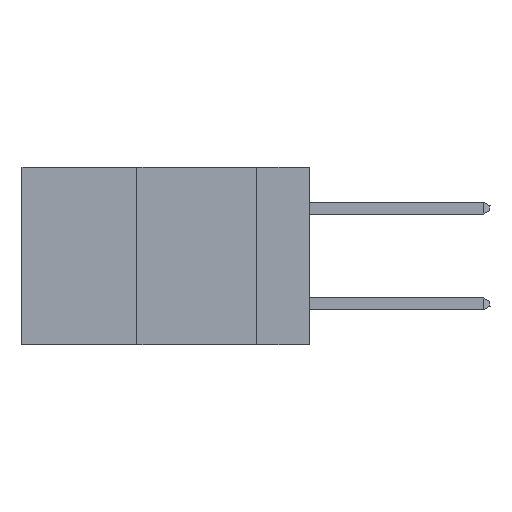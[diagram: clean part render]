
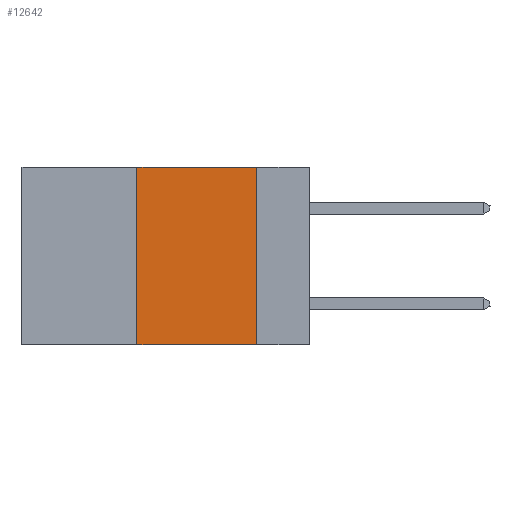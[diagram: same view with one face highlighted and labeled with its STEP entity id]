
A CAD part, left-side view. The second image highlights one B-rep face of the part: STEP entity #12642.
In plain terms, the highlighted planar face has unit normal (-1, 0, 0).
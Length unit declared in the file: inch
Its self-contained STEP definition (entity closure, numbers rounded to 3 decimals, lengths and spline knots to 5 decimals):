
#88 = CARTESIAN_POINT ( 'NONE',  ( 0., 0.36, 0. ) ) ;
#527 = CARTESIAN_POINT ( 'NONE',  ( 0., 0.6, 0. ) ) ;
#921 = LINE ( 'NONE', #35622, #24364 ) ;
#1566 = CARTESIAN_POINT ( 'NONE',  ( 0., 0.11, 0. ) ) ;
#4263 = EDGE_CURVE ( 'NONE', #24879, #12656, #921, .T. ) ;
#5585 = VECTOR ( 'NONE', #17706, 39.37008 ) ;
#6544 = LINE ( 'NONE', #11686, #5585 ) ;
#6609 = DIRECTION ( 'NONE',  ( 1., 0., 0. ) ) ;
#8636 = CARTESIAN_POINT ( 'NONE',  ( 0., 0.36, -0.37 ) ) ;
#8836 = LINE ( 'NONE', #35312, #28058 ) ;
#9610 = DIRECTION ( 'NONE',  ( 0., 0., -1. ) ) ;
#10953 = EDGE_CURVE ( 'NONE', #33151, #12656, #8836, .T. ) ;
#11686 = CARTESIAN_POINT ( 'NONE',  ( 0., 0.36, 0. ) ) ;
#11842 = ORIENTED_EDGE ( 'NONE', *, *, #33914, .F. ) ;
#12642 = ADVANCED_FACE ( 'NONE', ( #20418 ), #33520, .F. ) ;
#12656 = VERTEX_POINT ( 'NONE', #30481 ) ;
#14429 = DIRECTION ( 'NONE',  ( 0., -1., 0. ) ) ;
#15804 = VECTOR ( 'NONE', #14429, 39.37008 ) ;
#15939 = VERTEX_POINT ( 'NONE', #88 ) ;
#16555 = EDGE_CURVE ( 'NONE', #15939, #24879, #24757, .T. ) ;
#17706 = DIRECTION ( 'NONE',  ( 0., 0., 1. ) ) ;
#20418 = FACE_OUTER_BOUND ( 'NONE', #22758, .T. ) ;
#22758 = EDGE_LOOP ( 'NONE', ( #26031, #26876, #11842, #29586 ) ) ;
#24204 = DIRECTION ( 'NONE',  ( 0., -1., 0. ) ) ;
#24364 = VECTOR ( 'NONE', #29298, 39.37008 ) ;
#24757 = LINE ( 'NONE', #26315, #15804 ) ;
#24879 = VERTEX_POINT ( 'NONE', #1566 ) ;
#26031 = ORIENTED_EDGE ( 'NONE', *, *, #4263, .F. ) ;
#26315 = CARTESIAN_POINT ( 'NONE',  ( 0., 0.6, 0. ) ) ;
#26876 = ORIENTED_EDGE ( 'NONE', *, *, #16555, .F. ) ;
#28058 = VECTOR ( 'NONE', #24204, 39.37008 ) ;
#29298 = DIRECTION ( 'NONE',  ( 0., 0., -1. ) ) ;
#29586 = ORIENTED_EDGE ( 'NONE', *, *, #10953, .T. ) ;
#30481 = CARTESIAN_POINT ( 'NONE',  ( 0., 0.11, -0.37 ) ) ;
#33151 = VERTEX_POINT ( 'NONE', #8636 ) ;
#33520 = PLANE ( 'NONE',  #34024 ) ;
#33914 = EDGE_CURVE ( 'NONE', #33151, #15939, #6544, .T. ) ;
#34024 = AXIS2_PLACEMENT_3D ( 'NONE', #527, #6609, #9610 ) ;
#35312 = CARTESIAN_POINT ( 'NONE',  ( 0., 0.6, -0.37 ) ) ;
#35622 = CARTESIAN_POINT ( 'NONE',  ( 0., 0.11, 0. ) ) ;
